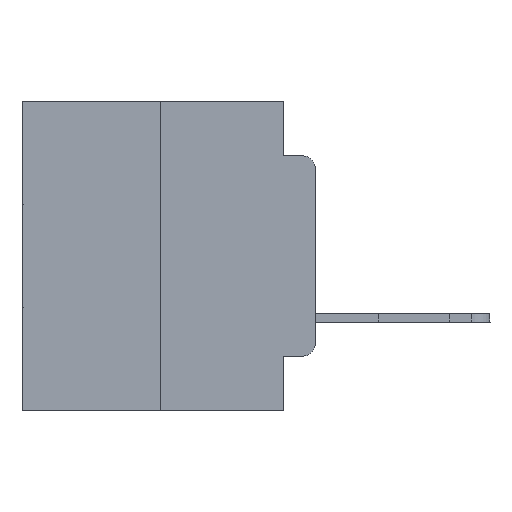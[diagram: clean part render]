
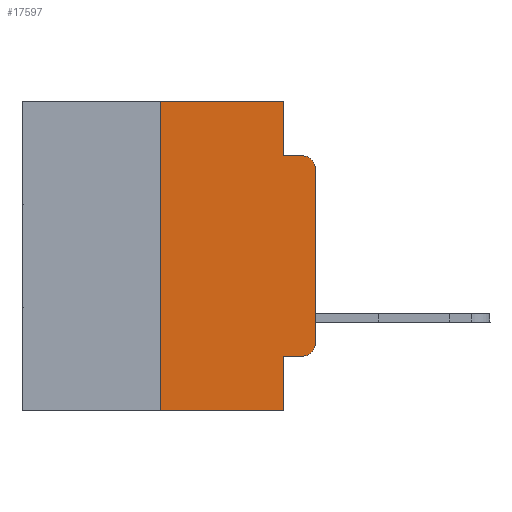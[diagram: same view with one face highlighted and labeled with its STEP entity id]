
A CAD part, left-side view. The second image highlights one B-rep face of the part: STEP entity #17597.
In plain terms, the highlighted planar face has unit normal (-1, 0, 0).
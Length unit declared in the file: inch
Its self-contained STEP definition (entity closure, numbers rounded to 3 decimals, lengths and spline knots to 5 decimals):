
#14 = ORIENTED_EDGE ( 'NONE', *, *, #17814, .F. ) ;
#191 = EDGE_CURVE ( 'NONE', #9320, #10252, #8622, .T. ) ;
#295 = DIRECTION ( 'NONE',  ( 0., 0., -1. ) ) ;
#1447 = DIRECTION ( 'NONE',  ( 0., 0., 1. ) ) ;
#2098 = VERTEX_POINT ( 'NONE', #17687 ) ;
#2152 = CIRCLE ( 'NONE', #12373, 0.02 ) ;
#2320 = CARTESIAN_POINT ( 'NONE',  ( 0., 0.051, 0. ) ) ;
#2344 = EDGE_CURVE ( 'NONE', #2858, #16714, #13942, .T. ) ;
#2657 = EDGE_CURVE ( 'NONE', #9320, #9473, #12558, .T. ) ;
#2858 = VERTEX_POINT ( 'NONE', #7007 ) ;
#3591 = VECTOR ( 'NONE', #6243, 39.37008 ) ;
#3861 = ORIENTED_EDGE ( 'NONE', *, *, #2344, .F. ) ;
#4141 = VECTOR ( 'NONE', #10918, 39.37008 ) ;
#4739 = ORIENTED_EDGE ( 'NONE', *, *, #6463, .T. ) ;
#5759 = CARTESIAN_POINT ( 'NONE',  ( 0., 0.25, 0. ) ) ;
#6243 = DIRECTION ( 'NONE',  ( 0., -1., 0. ) ) ;
#6463 = EDGE_CURVE ( 'NONE', #10252, #14681, #8677, .T. ) ;
#6529 = CARTESIAN_POINT ( 'NONE',  ( 0., 0.051, 0. ) ) ;
#6769 = VECTOR ( 'NONE', #22111, 39.37008 ) ;
#6870 = DIRECTION ( 'NONE',  ( 0., -1., 0. ) ) ;
#7007 = CARTESIAN_POINT ( 'NONE',  ( 0., 0.051, -0.0885 ) ) ;
#7326 = AXIS2_PLACEMENT_3D ( 'NONE', #9142, #13400, #295 ) ;
#7548 = EDGE_CURVE ( 'NONE', #26267, #9473, #12013, .T. ) ;
#7873 = EDGE_CURVE ( 'NONE', #14681, #25703, #16357, .T. ) ;
#8622 = LINE ( 'NONE', #26060, #19401 ) ;
#8677 = CIRCLE ( 'NONE', #7326, 0.02 ) ;
#8832 = CARTESIAN_POINT ( 'NONE',  ( 0., 0.25, 0. ) ) ;
#8974 = CARTESIAN_POINT ( 'NONE',  ( 0., 0.051, -0.5 ) ) ;
#9006 = FACE_OUTER_BOUND ( 'NONE', #11100, .T. ) ;
#9091 = ORIENTED_EDGE ( 'NONE', *, *, #15684, .T. ) ;
#9142 = CARTESIAN_POINT ( 'NONE',  ( 0., 0.02, -0.3915 ) ) ;
#9320 = VERTEX_POINT ( 'NONE', #22974 ) ;
#9473 = VERTEX_POINT ( 'NONE', #8974 ) ;
#10252 = VERTEX_POINT ( 'NONE', #23623 ) ;
#10918 = DIRECTION ( 'NONE',  ( 0., 0., -1. ) ) ;
#11100 = EDGE_LOOP ( 'NONE', ( #15949, #9091, #3861, #23981, #12346, #14, #27768, #23243, #25837, #4739 ) ) ;
#12013 = LINE ( 'NONE', #12838, #3591 ) ;
#12145 = VECTOR ( 'NONE', #24408, 39.37008 ) ;
#12346 = ORIENTED_EDGE ( 'NONE', *, *, #16669, .F. ) ;
#12373 = AXIS2_PLACEMENT_3D ( 'NONE', #27751, #27718, #15052 ) ;
#12558 = LINE ( 'NONE', #2320, #4141 ) ;
#12838 = CARTESIAN_POINT ( 'NONE',  ( 0., 0.473, -0.5 ) ) ;
#13037 = DIRECTION ( 'NONE',  ( 1., 0., 0. ) ) ;
#13400 = DIRECTION ( 'NONE',  ( -1., 0., 0. ) ) ;
#13942 = LINE ( 'NONE', #19934, #19949 ) ;
#14333 = DIRECTION ( 'NONE',  ( 0., 0., 1. ) ) ;
#14681 = VERTEX_POINT ( 'NONE', #24757 ) ;
#14948 = CARTESIAN_POINT ( 'NONE',  ( 0., 0., -0.1085 ) ) ;
#15052 = DIRECTION ( 'NONE',  ( 0., 0., -1. ) ) ;
#15684 = EDGE_CURVE ( 'NONE', #25703, #16714, #2152, .T. ) ;
#15949 = ORIENTED_EDGE ( 'NONE', *, *, #7873, .T. ) ;
#16357 = LINE ( 'NONE', #27342, #25768 ) ;
#16669 = EDGE_CURVE ( 'NONE', #27195, #2098, #18842, .T. ) ;
#16714 = VERTEX_POINT ( 'NONE', #25292 ) ;
#17597 = ADVANCED_FACE ( 'NONE', ( #9006 ), #17724, .F. ) ;
#17687 = CARTESIAN_POINT ( 'NONE',  ( 0., 0.051, 0. ) ) ;
#17724 = PLANE ( 'NONE',  #25002 ) ;
#17760 = CARTESIAN_POINT ( 'NONE',  ( 0., 0.473, 0. ) ) ;
#17814 = EDGE_CURVE ( 'NONE', #26267, #27195, #21441, .T. ) ;
#18268 = DIRECTION ( 'NONE',  ( 0., -1., 0. ) ) ;
#18842 = LINE ( 'NONE', #17760, #12145 ) ;
#19401 = VECTOR ( 'NONE', #6870, 39.37008 ) ;
#19934 = CARTESIAN_POINT ( 'NONE',  ( 0., 0.051, -0.0885 ) ) ;
#19949 = VECTOR ( 'NONE', #18268, 39.37008 ) ;
#21441 = LINE ( 'NONE', #5759, #27509 ) ;
#22111 = DIRECTION ( 'NONE',  ( 0., 0., -1. ) ) ;
#22974 = CARTESIAN_POINT ( 'NONE',  ( 0., 0.051, -0.4115 ) ) ;
#23243 = ORIENTED_EDGE ( 'NONE', *, *, #2657, .F. ) ;
#23623 = CARTESIAN_POINT ( 'NONE',  ( 0., 0.02, -0.4115 ) ) ;
#23927 = LINE ( 'NONE', #6529, #6769 ) ;
#23981 = ORIENTED_EDGE ( 'NONE', *, *, #27796, .F. ) ;
#24002 = CARTESIAN_POINT ( 'NONE',  ( 0., 0.25, -0.5 ) ) ;
#24183 = CARTESIAN_POINT ( 'NONE',  ( 0., 0.473, 0. ) ) ;
#24408 = DIRECTION ( 'NONE',  ( 0., -1., 0. ) ) ;
#24757 = CARTESIAN_POINT ( 'NONE',  ( 0., 0., -0.3915 ) ) ;
#25002 = AXIS2_PLACEMENT_3D ( 'NONE', #24183, #13037, #25992 ) ;
#25292 = CARTESIAN_POINT ( 'NONE',  ( 0., 0.02, -0.0885 ) ) ;
#25703 = VERTEX_POINT ( 'NONE', #14948 ) ;
#25768 = VECTOR ( 'NONE', #1447, 39.37008 ) ;
#25837 = ORIENTED_EDGE ( 'NONE', *, *, #191, .T. ) ;
#25992 = DIRECTION ( 'NONE',  ( 0., 0., -1. ) ) ;
#26060 = CARTESIAN_POINT ( 'NONE',  ( 0., 0.051, -0.4115 ) ) ;
#26267 = VERTEX_POINT ( 'NONE', #24002 ) ;
#27195 = VERTEX_POINT ( 'NONE', #8832 ) ;
#27342 = CARTESIAN_POINT ( 'NONE',  ( 0., 0., 0. ) ) ;
#27509 = VECTOR ( 'NONE', #14333, 39.37008 ) ;
#27718 = DIRECTION ( 'NONE',  ( -1., 0., 0. ) ) ;
#27751 = CARTESIAN_POINT ( 'NONE',  ( 0., 0.02, -0.1085 ) ) ;
#27768 = ORIENTED_EDGE ( 'NONE', *, *, #7548, .T. ) ;
#27796 = EDGE_CURVE ( 'NONE', #2098, #2858, #23927, .T. ) ;
